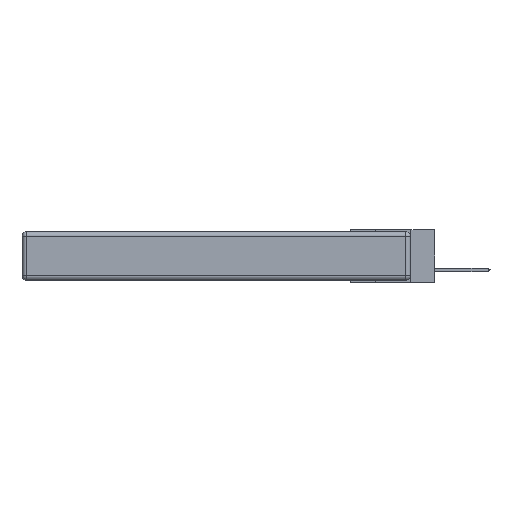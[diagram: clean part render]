
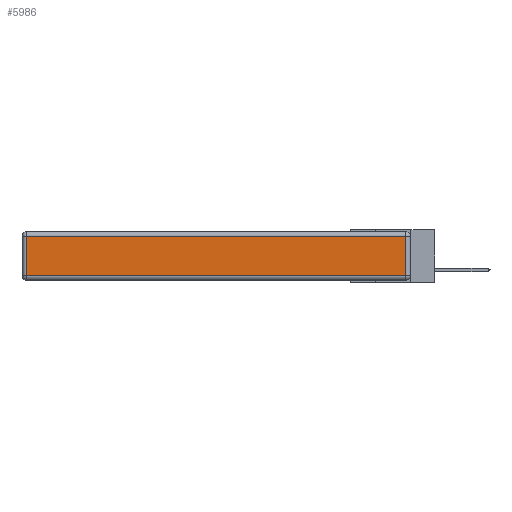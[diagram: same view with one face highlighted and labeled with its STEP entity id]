
A CAD part, left-side view. The second image highlights one B-rep face of the part: STEP entity #5986.
In plain terms, the highlighted planar face has unit normal (-1, 0, 0).
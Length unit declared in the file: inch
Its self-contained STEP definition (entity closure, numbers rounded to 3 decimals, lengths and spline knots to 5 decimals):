
#27 = VERTEX_POINT ( 'NONE', #4515 ) ;
#260 = CARTESIAN_POINT ( 'NONE',  ( 0., 2.72, -0.343 ) ) ;
#422 = CARTESIAN_POINT ( 'NONE',  ( 0., 0., -0.343 ) ) ;
#861 = LINE ( 'NONE', #260, #12714 ) ;
#881 = EDGE_LOOP ( 'NONE', ( #5286, #11177, #1994, #2078 ) ) ;
#1025 = CARTESIAN_POINT ( 'NONE',  ( 0., 2.72, -0.313 ) ) ;
#1368 = DIRECTION ( 'NONE',  ( 0., 0., 1. ) ) ;
#1482 = CARTESIAN_POINT ( 'NONE',  ( 0., 2.75, -0.03 ) ) ;
#1712 = LINE ( 'NONE', #1482, #11309 ) ;
#1994 = ORIENTED_EDGE ( 'NONE', *, *, #5036, .T. ) ;
#2078 = ORIENTED_EDGE ( 'NONE', *, *, #11574, .T. ) ;
#2386 = VECTOR ( 'NONE', #1368, 39.37008 ) ;
#2433 = DIRECTION ( 'NONE',  ( 0., 1., 0. ) ) ;
#2536 = CARTESIAN_POINT ( 'NONE',  ( 0., 0., -0.313 ) ) ;
#2637 = CARTESIAN_POINT ( 'NONE',  ( 0., 0.03, -0.313 ) ) ;
#3418 = EDGE_CURVE ( 'NONE', #6012, #10809, #11026, .T. ) ;
#3456 = CARTESIAN_POINT ( 'NONE',  ( 0., 0.03, -0.03 ) ) ;
#3526 = CARTESIAN_POINT ( 'NONE',  ( 0., 0.03, -0.343 ) ) ;
#4515 = CARTESIAN_POINT ( 'NONE',  ( 0., 2.72, -0.03 ) ) ;
#4658 = PLANE ( 'NONE',  #8095 ) ;
#5036 = EDGE_CURVE ( 'NONE', #10809, #27, #1712, .T. ) ;
#5286 = ORIENTED_EDGE ( 'NONE', *, *, #12399, .T. ) ;
#5986 = ADVANCED_FACE ( 'NONE', ( #12715 ), #4658, .T. ) ;
#6012 = VERTEX_POINT ( 'NONE', #2637 ) ;
#7776 = DIRECTION ( 'NONE',  ( -1., 0., 0. ) ) ;
#7792 = VERTEX_POINT ( 'NONE', #1025 ) ;
#8095 = AXIS2_PLACEMENT_3D ( 'NONE', #422, #7776, #12835 ) ;
#8500 = DIRECTION ( 'NONE',  ( 0., 0., -1. ) ) ;
#9675 = DIRECTION ( 'NONE',  ( 0., -1., 0. ) ) ;
#9978 = VECTOR ( 'NONE', #9675, 39.37008 ) ;
#10809 = VERTEX_POINT ( 'NONE', #3456 ) ;
#11026 = LINE ( 'NONE', #3526, #2386 ) ;
#11177 = ORIENTED_EDGE ( 'NONE', *, *, #3418, .T. ) ;
#11309 = VECTOR ( 'NONE', #2433, 39.37008 ) ;
#11574 = EDGE_CURVE ( 'NONE', #27, #7792, #861, .T. ) ;
#12399 = EDGE_CURVE ( 'NONE', #7792, #6012, #12846, .T. ) ;
#12714 = VECTOR ( 'NONE', #8500, 39.37008 ) ;
#12715 = FACE_OUTER_BOUND ( 'NONE', #881, .T. ) ;
#12835 = DIRECTION ( 'NONE',  ( 0., 0., 1. ) ) ;
#12846 = LINE ( 'NONE', #2536, #9978 ) ;
